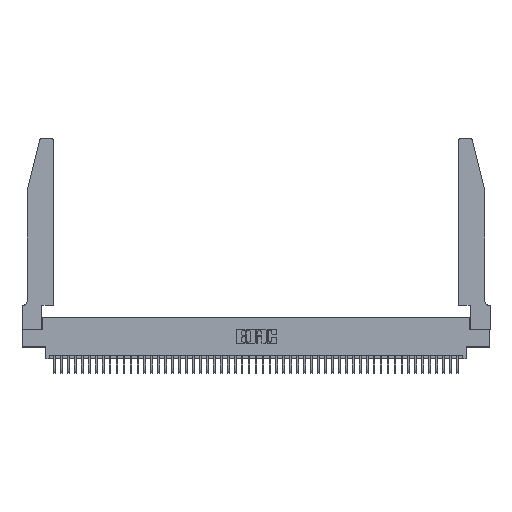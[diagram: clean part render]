
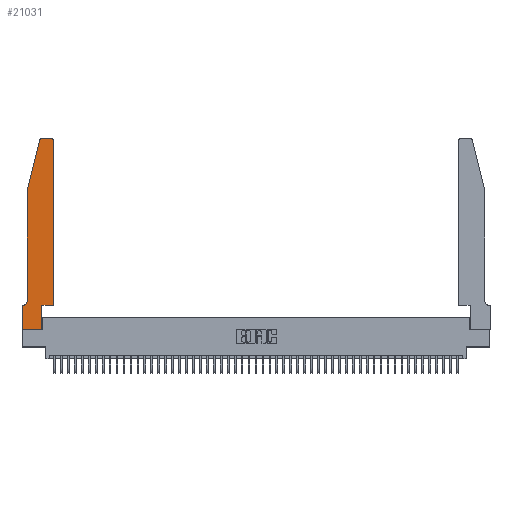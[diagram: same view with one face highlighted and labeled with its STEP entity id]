
A CAD part, top view. The second image highlights one B-rep face of the part: STEP entity #21031.
In plain terms, the highlighted planar face has unit normal (0, 0, 1).
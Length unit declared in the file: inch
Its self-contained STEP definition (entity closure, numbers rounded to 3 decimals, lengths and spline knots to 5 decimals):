
#476 = EDGE_CURVE ( 'NONE', #6624, #3317, #837, .T. ) ;
#666 = DIRECTION ( 'NONE',  ( 0., 1., 0. ) ) ;
#713 = DIRECTION ( 'NONE',  ( -1., 0., 0. ) ) ;
#837 = LINE ( 'NONE', #16863, #28434 ) ;
#2004 = ORIENTED_EDGE ( 'NONE', *, *, #476, .T. ) ;
#2333 = AXIS2_PLACEMENT_3D ( 'NONE', #36459, #28536, #12419 ) ;
#3025 = LINE ( 'NONE', #50338, #4847 ) ;
#3113 = CARTESIAN_POINT ( 'NONE',  ( 0.4505, 0.35, 0.37 ) ) ;
#3317 = VERTEX_POINT ( 'NONE', #40935 ) ;
#4016 = VECTOR ( 'NONE', #21263, 39.37008 ) ;
#4099 = CARTESIAN_POINT ( 'NONE',  ( 0.4505, 0.35, 0.37 ) ) ;
#4847 = VECTOR ( 'NONE', #46373, 39.37008 ) ;
#4882 = EDGE_CURVE ( 'NONE', #41889, #6624, #29787, .T. ) ;
#5118 = PLANE ( 'NONE',  #47855 ) ;
#6624 = VERTEX_POINT ( 'NONE', #47936 ) ;
#7141 = VERTEX_POINT ( 'NONE', #35978 ) ;
#7225 = ORIENTED_EDGE ( 'NONE', *, *, #9257, .T. ) ;
#9257 = EDGE_CURVE ( 'NONE', #49488, #7141, #43403, .T. ) ;
#9623 = EDGE_CURVE ( 'NONE', #40330, #13816, #3025, .T. ) ;
#9725 = DIRECTION ( 'NONE',  ( -1., 0., 0. ) ) ;
#9884 = EDGE_CURVE ( 'NONE', #7141, #41889, #25033, .T. ) ;
#10760 = CARTESIAN_POINT ( 'NONE',  ( 0.4505, 2.72, 0.37 ) ) ;
#10771 = LINE ( 'NONE', #13724, #4016 ) ;
#11233 = CARTESIAN_POINT ( 'NONE',  ( 0.0055, 0.42, 0.37 ) ) ;
#12031 = EDGE_CURVE ( 'NONE', #3317, #19748, #30629, .T. ) ;
#12419 = DIRECTION ( 'NONE',  ( 1., 0., 0. ) ) ;
#13204 = EDGE_CURVE ( 'NONE', #13816, #34342, #13966, .T. ) ;
#13724 = CARTESIAN_POINT ( 'NONE',  ( 0., 0., 0.37 ) ) ;
#13816 = VERTEX_POINT ( 'NONE', #41251 ) ;
#13909 = ORIENTED_EDGE ( 'NONE', *, *, #13204, .T. ) ;
#13966 = LINE ( 'NONE', #45049, #49330 ) ;
#16213 = ORIENTED_EDGE ( 'NONE', *, *, #49645, .T. ) ;
#16248 = EDGE_LOOP ( 'NONE', ( #7225, #42434, #34857, #2004, #40320, #27842, #45804, #39339, #13909, #16213, #49050, #39219 ) ) ;
#16843 = CIRCLE ( 'NONE', #2333, 0.03 ) ;
#16863 = CARTESIAN_POINT ( 'NONE',  ( 0.0755, 2., 0.37 ) ) ;
#17515 = DIRECTION ( 'NONE',  ( 1., 0., 0. ) ) ;
#17983 = VERTEX_POINT ( 'NONE', #3113 ) ;
#18089 = CARTESIAN_POINT ( 'NONE',  ( 0.25487, 2.72718, 0.37 ) ) ;
#19748 = VERTEX_POINT ( 'NONE', #30844 ) ;
#20540 = VECTOR ( 'NONE', #666, 39.37008 ) ;
#20629 = CARTESIAN_POINT ( 'NONE',  ( 0., 0., 0.37 ) ) ;
#20812 = VECTOR ( 'NONE', #713, 39.37008 ) ;
#20820 = DIRECTION ( 'NONE',  ( 0., -1., 0. ) ) ;
#20866 = DIRECTION ( 'NONE',  ( 1., 0., 0. ) ) ;
#21031 = ADVANCED_FACE ( 'NONE', ( #49082 ), #5118, .T. ) ;
#21263 = DIRECTION ( 'NONE',  ( 0., -1., 0. ) ) ;
#21744 = DIRECTION ( 'NONE',  ( 0., 1., 0. ) ) ;
#23211 = DIRECTION ( 'NONE',  ( -1., 0., 0. ) ) ;
#24302 = CARTESIAN_POINT ( 'NONE',  ( 0.0755, 2., 0.37 ) ) ;
#24877 = CARTESIAN_POINT ( 'NONE',  ( 0.4205, 2.75, 0.37 ) ) ;
#25033 = CIRCLE ( 'NONE', #28698, 0.03 ) ;
#25449 = CARTESIAN_POINT ( 'NONE',  ( 0.0755, 0.35, 0.37 ) ) ;
#27231 = DIRECTION ( 'NONE',  ( 0., 0., 1. ) ) ;
#27725 = LINE ( 'NONE', #41190, #49556 ) ;
#27825 = VERTEX_POINT ( 'NONE', #10760 ) ;
#27842 = ORIENTED_EDGE ( 'NONE', *, *, #45122, .T. ) ;
#28085 = DIRECTION ( 'NONE',  ( -0.239, -0.971, 0. ) ) ;
#28434 = VECTOR ( 'NONE', #20820, 39.37008 ) ;
#28536 = DIRECTION ( 'NONE',  ( 0., 0., 1. ) ) ;
#28698 = AXIS2_PLACEMENT_3D ( 'NONE', #50509, #27231, #35025 ) ;
#29787 = LINE ( 'NONE', #24302, #34646 ) ;
#30629 = CIRCLE ( 'NONE', #44384, 0.07 ) ;
#30844 = CARTESIAN_POINT ( 'NONE',  ( 0.0055, 0.35, 0.37 ) ) ;
#31332 = CARTESIAN_POINT ( 'NONE',  ( 0.2865, 0.35, 0.37 ) ) ;
#32472 = CARTESIAN_POINT ( 'NONE',  ( 0., 0.35, 0.37 ) ) ;
#34299 = DIRECTION ( 'NONE',  ( 0., 0., -1. ) ) ;
#34342 = VERTEX_POINT ( 'NONE', #31332 ) ;
#34646 = VECTOR ( 'NONE', #28085, 39.37008 ) ;
#34857 = ORIENTED_EDGE ( 'NONE', *, *, #4882, .T. ) ;
#34914 = CARTESIAN_POINT ( 'NONE',  ( 0.2605, 2.75, 0.37 ) ) ;
#35025 = DIRECTION ( 'NONE',  ( 1., 0., 0. ) ) ;
#35978 = CARTESIAN_POINT ( 'NONE',  ( 0.284, 2.75, 0.37 ) ) ;
#36459 = CARTESIAN_POINT ( 'NONE',  ( 0.4205, 2.72, 0.37 ) ) ;
#37370 = EDGE_CURVE ( 'NONE', #27825, #49488, #16843, .T. ) ;
#39219 = ORIENTED_EDGE ( 'NONE', *, *, #37370, .T. ) ;
#39339 = ORIENTED_EDGE ( 'NONE', *, *, #9623, .T. ) ;
#40320 = ORIENTED_EDGE ( 'NONE', *, *, #12031, .T. ) ;
#40330 = VERTEX_POINT ( 'NONE', #20629 ) ;
#40844 = VECTOR ( 'NONE', #9725, 39.37008 ) ;
#40935 = CARTESIAN_POINT ( 'NONE',  ( 0.0755, 0.42, 0.37 ) ) ;
#41190 = CARTESIAN_POINT ( 'NONE',  ( 0.4505, 0.35, 0.37 ) ) ;
#41251 = CARTESIAN_POINT ( 'NONE',  ( 0.2865, 0., 0.37 ) ) ;
#41842 = LINE ( 'NONE', #4099, #20540 ) ;
#41889 = VERTEX_POINT ( 'NONE', #18089 ) ;
#42434 = ORIENTED_EDGE ( 'NONE', *, *, #9884, .T. ) ;
#43305 = LINE ( 'NONE', #25449, #40844 ) ;
#43403 = LINE ( 'NONE', #34914, #20812 ) ;
#44198 = DIRECTION ( 'NONE',  ( 0., 0., 1. ) ) ;
#44384 = AXIS2_PLACEMENT_3D ( 'NONE', #11233, #34299, #23211 ) ;
#45049 = CARTESIAN_POINT ( 'NONE',  ( 0.2865, 0.35, 0.37 ) ) ;
#45122 = EDGE_CURVE ( 'NONE', #19748, #45490, #43305, .T. ) ;
#45233 = CARTESIAN_POINT ( 'NONE',  ( 0., 0.35, 0.37 ) ) ;
#45490 = VERTEX_POINT ( 'NONE', #45233 ) ;
#45804 = ORIENTED_EDGE ( 'NONE', *, *, #47390, .T. ) ;
#46373 = DIRECTION ( 'NONE',  ( 1., 0., 0. ) ) ;
#47390 = EDGE_CURVE ( 'NONE', #45490, #40330, #10771, .T. ) ;
#47780 = EDGE_CURVE ( 'NONE', #17983, #27825, #41842, .T. ) ;
#47855 = AXIS2_PLACEMENT_3D ( 'NONE', #32472, #44198, #20866 ) ;
#47936 = CARTESIAN_POINT ( 'NONE',  ( 0.0755, 2., 0.37 ) ) ;
#49050 = ORIENTED_EDGE ( 'NONE', *, *, #47780, .T. ) ;
#49082 = FACE_OUTER_BOUND ( 'NONE', #16248, .T. ) ;
#49330 = VECTOR ( 'NONE', #21744, 39.37008 ) ;
#49488 = VERTEX_POINT ( 'NONE', #24877 ) ;
#49556 = VECTOR ( 'NONE', #17515, 39.37008 ) ;
#49645 = EDGE_CURVE ( 'NONE', #34342, #17983, #27725, .T. ) ;
#50338 = CARTESIAN_POINT ( 'NONE',  ( 0., 0., 0.37 ) ) ;
#50509 = CARTESIAN_POINT ( 'NONE',  ( 0.284, 2.72, 0.37 ) ) ;
